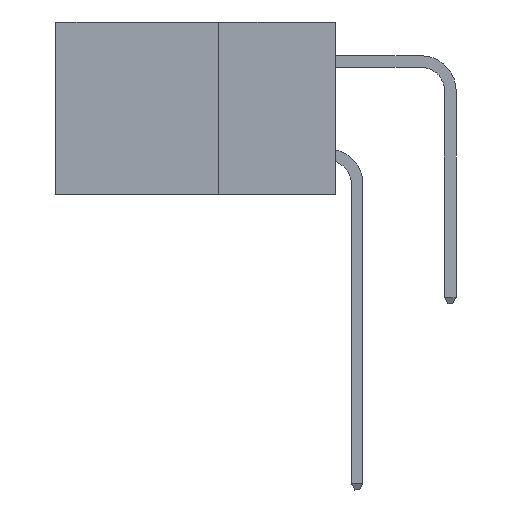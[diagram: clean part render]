
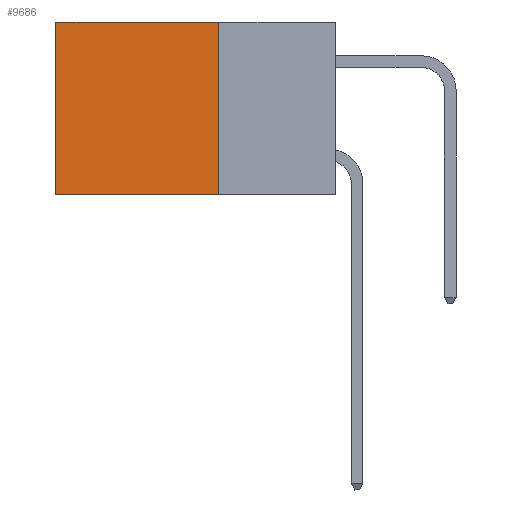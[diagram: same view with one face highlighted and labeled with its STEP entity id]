
A CAD part, left-side view. The second image highlights one B-rep face of the part: STEP entity #9686.
In plain terms, the highlighted planar face has unit normal (-1, 0, 0).
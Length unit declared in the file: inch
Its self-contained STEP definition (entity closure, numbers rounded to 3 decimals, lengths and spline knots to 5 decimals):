
#442 = LINE ( 'NONE', #5651, #6559 ) ;
#2543 = CARTESIAN_POINT ( 'NONE',  ( 0.2875, 0.25, 0. ) ) ;
#3750 = AXIS2_PLACEMENT_3D ( 'NONE', #21255, #23145, #21089 ) ;
#4014 = DIRECTION ( 'NONE',  ( 0., 1., 0. ) ) ;
#4798 = CARTESIAN_POINT ( 'NONE',  ( 0.2875, 0.25, -0.37 ) ) ;
#5651 = CARTESIAN_POINT ( 'NONE',  ( 0.2875, 0.25, 0. ) ) ;
#5892 = CARTESIAN_POINT ( 'NONE',  ( 0.2875, 0.6, -0.37 ) ) ;
#6559 = VECTOR ( 'NONE', #11286, 39.37008 ) ;
#6674 = LINE ( 'NONE', #2543, #12237 ) ;
#6877 = VERTEX_POINT ( 'NONE', #4798 ) ;
#7199 = EDGE_LOOP ( 'NONE', ( #19555, #14849, #8244, #19229 ) ) ;
#7285 = EDGE_CURVE ( 'NONE', #13199, #17368, #13080, .T. ) ;
#7820 = CARTESIAN_POINT ( 'NONE',  ( 0.2875, 0.6, 0. ) ) ;
#7973 = VERTEX_POINT ( 'NONE', #17153 ) ;
#8119 = VECTOR ( 'NONE', #20917, 39.37008 ) ;
#8244 = ORIENTED_EDGE ( 'NONE', *, *, #9468, .F. ) ;
#9468 = EDGE_CURVE ( 'NONE', #7973, #6877, #442, .T. ) ;
#9686 = ADVANCED_FACE ( 'NONE', ( #11499 ), #17541, .F. ) ;
#10287 = VECTOR ( 'NONE', #4014, 39.37008 ) ;
#11286 = DIRECTION ( 'NONE',  ( 0., 0., -1. ) ) ;
#11499 = FACE_OUTER_BOUND ( 'NONE', #7199, .T. ) ;
#12237 = VECTOR ( 'NONE', #15608, 39.37008 ) ;
#13080 = LINE ( 'NONE', #7820, #8119 ) ;
#13199 = VERTEX_POINT ( 'NONE', #22478 ) ;
#14849 = ORIENTED_EDGE ( 'NONE', *, *, #22309, .F. ) ;
#15038 = CARTESIAN_POINT ( 'NONE',  ( 0.2875, 0.25, -0.37 ) ) ;
#15608 = DIRECTION ( 'NONE',  ( 0., 1., 0. ) ) ;
#16723 = LINE ( 'NONE', #15038, #10287 ) ;
#17153 = CARTESIAN_POINT ( 'NONE',  ( 0.2875, 0.25, 0. ) ) ;
#17368 = VERTEX_POINT ( 'NONE', #5892 ) ;
#17541 = PLANE ( 'NONE',  #3750 ) ;
#19229 = ORIENTED_EDGE ( 'NONE', *, *, #24200, .T. ) ;
#19555 = ORIENTED_EDGE ( 'NONE', *, *, #7285, .T. ) ;
#20917 = DIRECTION ( 'NONE',  ( 0., 0., -1. ) ) ;
#21089 = DIRECTION ( 'NONE',  ( 0., 0., -1. ) ) ;
#21255 = CARTESIAN_POINT ( 'NONE',  ( 0.2875, 0.25, 0. ) ) ;
#22309 = EDGE_CURVE ( 'NONE', #6877, #17368, #16723, .T. ) ;
#22478 = CARTESIAN_POINT ( 'NONE',  ( 0.2875, 0.6, 0. ) ) ;
#23145 = DIRECTION ( 'NONE',  ( 1., 0., 0. ) ) ;
#24200 = EDGE_CURVE ( 'NONE', #7973, #13199, #6674, .T. ) ;
